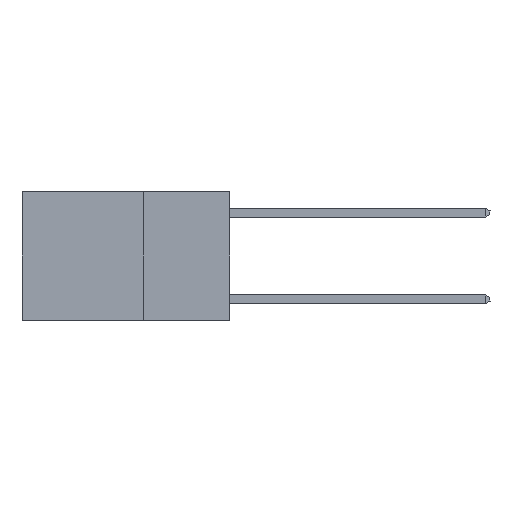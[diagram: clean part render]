
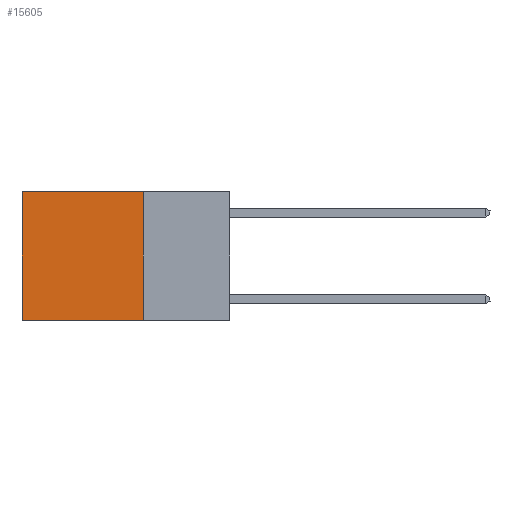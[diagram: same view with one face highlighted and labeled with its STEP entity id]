
A CAD part, left-side view. The second image highlights one B-rep face of the part: STEP entity #15605.
In plain terms, the highlighted planar face has unit normal (-1, 0, 0).
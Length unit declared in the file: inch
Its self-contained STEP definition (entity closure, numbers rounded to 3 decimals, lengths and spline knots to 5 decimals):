
#1134 = VECTOR ( 'NONE', #12464, 39.37008 ) ;
#1206 = AXIS2_PLACEMENT_3D ( 'NONE', #10287, #14143, #14321 ) ;
#1855 = CARTESIAN_POINT ( 'NONE',  ( 0.2625, 0.25, 0. ) ) ;
#2257 = EDGE_CURVE ( 'NONE', #15567, #8713, #16692, .T. ) ;
#2804 = CARTESIAN_POINT ( 'NONE',  ( 0.2625, 0.6, 0. ) ) ;
#2946 = CARTESIAN_POINT ( 'NONE',  ( 0.2625, 0.25, 0. ) ) ;
#3559 = CARTESIAN_POINT ( 'NONE',  ( 0.2625, 0.25, -0.37 ) ) ;
#3681 = VERTEX_POINT ( 'NONE', #2946 ) ;
#3747 = CARTESIAN_POINT ( 'NONE',  ( 0.2625, 0.6, 0. ) ) ;
#4843 = PLANE ( 'NONE',  #1206 ) ;
#5567 = LINE ( 'NONE', #1855, #17036 ) ;
#5573 = EDGE_CURVE ( 'NONE', #3681, #6912, #5567, .T. ) ;
#5678 = DIRECTION ( 'NONE',  ( 0., 1., 0. ) ) ;
#6225 = VECTOR ( 'NONE', #7407, 39.37008 ) ;
#6326 = DIRECTION ( 'NONE',  ( 0., 0., -1. ) ) ;
#6858 = ORIENTED_EDGE ( 'NONE', *, *, #13227, .F. ) ;
#6912 = VERTEX_POINT ( 'NONE', #2804 ) ;
#7072 = LINE ( 'NONE', #3747, #17077 ) ;
#7407 = DIRECTION ( 'NONE',  ( 0., 1., 0. ) ) ;
#8713 = VERTEX_POINT ( 'NONE', #16277 ) ;
#8771 = LINE ( 'NONE', #10479, #1134 ) ;
#9486 = ORIENTED_EDGE ( 'NONE', *, *, #5573, .T. ) ;
#9972 = EDGE_LOOP ( 'NONE', ( #13526, #16007, #6858, #9486 ) ) ;
#10287 = CARTESIAN_POINT ( 'NONE',  ( 0.2625, 0.25, 0. ) ) ;
#10479 = CARTESIAN_POINT ( 'NONE',  ( 0.2625, 0.25, 0. ) ) ;
#12270 = FACE_OUTER_BOUND ( 'NONE', #9972, .T. ) ;
#12464 = DIRECTION ( 'NONE',  ( 0., 0., -1. ) ) ;
#12856 = CARTESIAN_POINT ( 'NONE',  ( 0.2625, 0.25, -0.37 ) ) ;
#13227 = EDGE_CURVE ( 'NONE', #3681, #15567, #8771, .T. ) ;
#13526 = ORIENTED_EDGE ( 'NONE', *, *, #15556, .T. ) ;
#14143 = DIRECTION ( 'NONE',  ( 1., 0., 0. ) ) ;
#14321 = DIRECTION ( 'NONE',  ( 0., 0., -1. ) ) ;
#15556 = EDGE_CURVE ( 'NONE', #6912, #8713, #7072, .T. ) ;
#15567 = VERTEX_POINT ( 'NONE', #12856 ) ;
#15605 = ADVANCED_FACE ( 'NONE', ( #12270 ), #4843, .F. ) ;
#16007 = ORIENTED_EDGE ( 'NONE', *, *, #2257, .F. ) ;
#16277 = CARTESIAN_POINT ( 'NONE',  ( 0.2625, 0.6, -0.37 ) ) ;
#16692 = LINE ( 'NONE', #3559, #6225 ) ;
#17036 = VECTOR ( 'NONE', #5678, 39.37008 ) ;
#17077 = VECTOR ( 'NONE', #6326, 39.37008 ) ;
